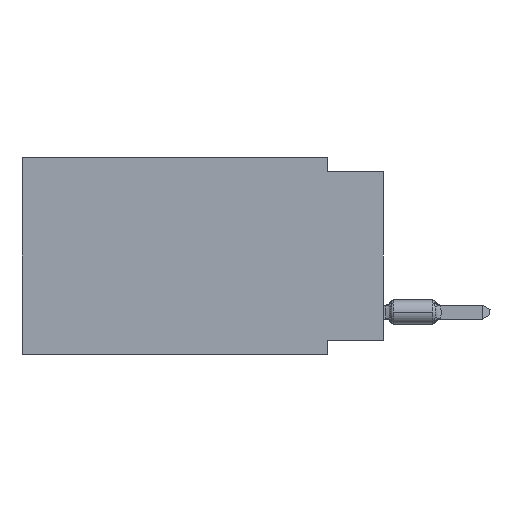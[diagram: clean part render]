
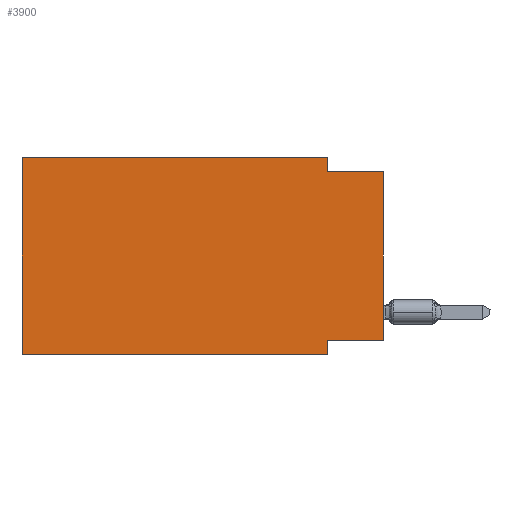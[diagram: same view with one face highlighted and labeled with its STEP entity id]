
A CAD part, left-side view. The second image highlights one B-rep face of the part: STEP entity #3900.
In plain terms, the highlighted planar face has unit normal (-1, 0, 0).
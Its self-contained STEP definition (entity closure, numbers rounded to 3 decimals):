
#213 = PLANE ( 'NONE',  #31415 ) ;
#296 = DIRECTION ( 'NONE',  ( 0., 0., -1. ) ) ;
#418 = EDGE_CURVE ( 'NONE', #25174, #2084, #34160, .T. ) ;
#720 = CARTESIAN_POINT ( 'NONE',  ( 0., 0., -0.635 ) ) ;
#1002 = VECTOR ( 'NONE', #5932, 1000. ) ;
#1471 = CARTESIAN_POINT ( 'NONE',  ( 0., 2.54, -0.635 ) ) ;
#2084 = VERTEX_POINT ( 'NONE', #6793 ) ;
#2643 = EDGE_CURVE ( 'NONE', #25174, #33260, #7213, .T. ) ;
#2690 = DIRECTION ( 'NONE',  ( 0., 1., 0. ) ) ;
#3900 = ADVANCED_FACE ( 'NONE', ( #8743 ), #213, .F. ) ;
#5932 = DIRECTION ( 'NONE',  ( 0., -1., 0. ) ) ;
#6231 = CARTESIAN_POINT ( 'NONE',  ( 0., 2.54, -8.89 ) ) ;
#6330 = DIRECTION ( 'NONE',  ( 0., 0., -1. ) ) ;
#6589 = EDGE_CURVE ( 'NONE', #33260, #23887, #11769, .T. ) ;
#6793 = CARTESIAN_POINT ( 'NONE',  ( 0., 2.54, -8.89 ) ) ;
#6807 = ORIENTED_EDGE ( 'NONE', *, *, #418, .T. ) ;
#7034 = VECTOR ( 'NONE', #2690, 1000. ) ;
#7213 = LINE ( 'NONE', #24643, #34257 ) ;
#8473 = EDGE_LOOP ( 'NONE', ( #10315, #32411, #32356, #25886, #23409, #6807, #29800, #17629 ) ) ;
#8743 = FACE_OUTER_BOUND ( 'NONE', #8473, .T. ) ;
#8757 = DIRECTION ( 'NONE',  ( 0., -1., 0. ) ) ;
#8925 = LINE ( 'NONE', #23382, #23157 ) ;
#8932 = DIRECTION ( 'NONE',  ( 1., 0., 0. ) ) ;
#9082 = CARTESIAN_POINT ( 'NONE',  ( 0., 2.54, -8.255 ) ) ;
#9339 = VECTOR ( 'NONE', #13469, 1000. ) ;
#10168 = CARTESIAN_POINT ( 'NONE',  ( 0., 0., -0.635 ) ) ;
#10315 = ORIENTED_EDGE ( 'NONE', *, *, #34788, .T. ) ;
#11712 = VERTEX_POINT ( 'NONE', #1471 ) ;
#11769 = LINE ( 'NONE', #34923, #19142 ) ;
#12050 = LINE ( 'NONE', #720, #1002 ) ;
#12071 = CARTESIAN_POINT ( 'NONE',  ( 0., 0., -8.255 ) ) ;
#13093 = EDGE_CURVE ( 'NONE', #23887, #11712, #28100, .T. ) ;
#13469 = DIRECTION ( 'NONE',  ( 0., 0., -1. ) ) ;
#15534 = VERTEX_POINT ( 'NONE', #10168 ) ;
#16617 = CARTESIAN_POINT ( 'NONE',  ( 0., 2.54, 0. ) ) ;
#17505 = LINE ( 'NONE', #28826, #7034 ) ;
#17629 = ORIENTED_EDGE ( 'NONE', *, *, #26598, .F. ) ;
#18913 = VERTEX_POINT ( 'NONE', #12071 ) ;
#19142 = VECTOR ( 'NONE', #34553, 1000. ) ;
#20052 = CARTESIAN_POINT ( 'NONE',  ( 0., 16.383, 0. ) ) ;
#20066 = CARTESIAN_POINT ( 'NONE',  ( 0., 16.383, -8.89 ) ) ;
#21300 = DIRECTION ( 'NONE',  ( 0., 0., 1. ) ) ;
#21367 = VERTEX_POINT ( 'NONE', #9082 ) ;
#22342 = CARTESIAN_POINT ( 'NONE',  ( 0., 2.54, 0. ) ) ;
#23157 = VECTOR ( 'NONE', #25615, 1000. ) ;
#23382 = CARTESIAN_POINT ( 'NONE',  ( 0., 0., 0. ) ) ;
#23409 = ORIENTED_EDGE ( 'NONE', *, *, #2643, .F. ) ;
#23887 = VERTEX_POINT ( 'NONE', #16617 ) ;
#24643 = CARTESIAN_POINT ( 'NONE',  ( 0., 16.383, 0. ) ) ;
#24658 = CARTESIAN_POINT ( 'NONE',  ( 0., 16.383, -8.89 ) ) ;
#25174 = VERTEX_POINT ( 'NONE', #24658 ) ;
#25615 = DIRECTION ( 'NONE',  ( 0., 0., 1. ) ) ;
#25686 = EDGE_CURVE ( 'NONE', #11712, #15534, #12050, .T. ) ;
#25884 = LINE ( 'NONE', #6231, #32066 ) ;
#25886 = ORIENTED_EDGE ( 'NONE', *, *, #6589, .F. ) ;
#26375 = CARTESIAN_POINT ( 'NONE',  ( 0., 16.383, 0. ) ) ;
#26598 = EDGE_CURVE ( 'NONE', #18913, #21367, #17505, .T. ) ;
#28100 = LINE ( 'NONE', #22342, #9339 ) ;
#28826 = CARTESIAN_POINT ( 'NONE',  ( 0., 0., -8.255 ) ) ;
#29800 = ORIENTED_EDGE ( 'NONE', *, *, #35563, .F. ) ;
#31415 = AXIS2_PLACEMENT_3D ( 'NONE', #20052, #8932, #6330 ) ;
#32066 = VECTOR ( 'NONE', #296, 1000. ) ;
#32356 = ORIENTED_EDGE ( 'NONE', *, *, #13093, .F. ) ;
#32411 = ORIENTED_EDGE ( 'NONE', *, *, #25686, .F. ) ;
#33260 = VERTEX_POINT ( 'NONE', #26375 ) ;
#33656 = VECTOR ( 'NONE', #8757, 1000. ) ;
#34160 = LINE ( 'NONE', #20066, #33656 ) ;
#34257 = VECTOR ( 'NONE', #21300, 1000. ) ;
#34553 = DIRECTION ( 'NONE',  ( 0., -1., 0. ) ) ;
#34788 = EDGE_CURVE ( 'NONE', #18913, #15534, #8925, .T. ) ;
#34923 = CARTESIAN_POINT ( 'NONE',  ( 0., 16.383, 0. ) ) ;
#35563 = EDGE_CURVE ( 'NONE', #21367, #2084, #25884, .T. ) ;
